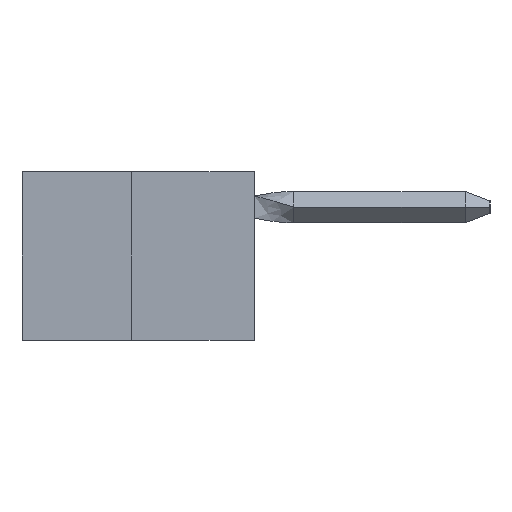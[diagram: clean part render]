
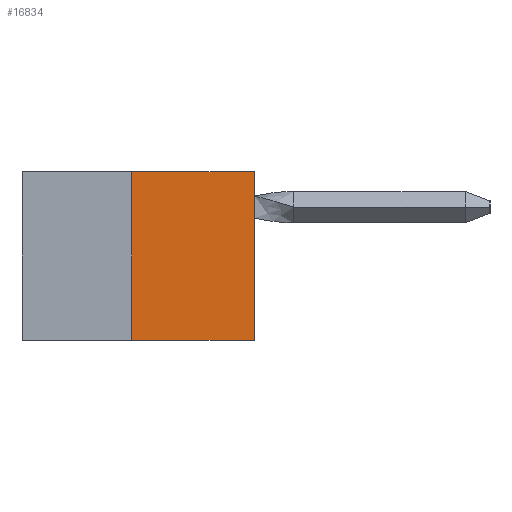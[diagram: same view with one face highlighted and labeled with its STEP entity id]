
A CAD part, left-side view. The second image highlights one B-rep face of the part: STEP entity #16834.
In plain terms, the highlighted planar face has unit normal (-1, 0, 0).
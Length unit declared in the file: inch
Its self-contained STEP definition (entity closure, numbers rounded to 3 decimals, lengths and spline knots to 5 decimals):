
#616 = DIRECTION ( 'NONE',  ( 0., 0., -1. ) ) ;
#1015 = CARTESIAN_POINT ( 'NONE',  ( 0., 0.473, -0.343 ) ) ;
#1435 = VERTEX_POINT ( 'NONE', #10154 ) ;
#1439 = EDGE_CURVE ( 'NONE', #32451, #29499, #21421, .T. ) ;
#4419 = VERTEX_POINT ( 'NONE', #32330 ) ;
#4505 = VECTOR ( 'NONE', #20244, 39.37008 ) ;
#6474 = LINE ( 'NONE', #13407, #26571 ) ;
#6971 = CARTESIAN_POINT ( 'NONE',  ( 0., 0.25, 0. ) ) ;
#7563 = VECTOR ( 'NONE', #35632, 39.37008 ) ;
#8974 = ORIENTED_EDGE ( 'NONE', *, *, #36058, .T. ) ;
#8975 = CARTESIAN_POINT ( 'NONE',  ( 0., 0.473, 0. ) ) ;
#10154 = CARTESIAN_POINT ( 'NONE',  ( 0., 0., 0. ) ) ;
#11006 = LINE ( 'NONE', #1015, #36489 ) ;
#12723 = CARTESIAN_POINT ( 'NONE',  ( 0., 0.25, -0.343 ) ) ;
#13407 = CARTESIAN_POINT ( 'NONE',  ( 0., 0., 0. ) ) ;
#13809 = AXIS2_PLACEMENT_3D ( 'NONE', #8975, #34700, #616 ) ;
#14290 = ORIENTED_EDGE ( 'NONE', *, *, #31448, .T. ) ;
#14759 = CARTESIAN_POINT ( 'NONE',  ( 0., 0.473, 0. ) ) ;
#16834 = ADVANCED_FACE ( 'NONE', ( #19210 ), #29084, .F. ) ;
#19210 = FACE_OUTER_BOUND ( 'NONE', #25173, .T. ) ;
#20244 = DIRECTION ( 'NONE',  ( 0., -1., 0. ) ) ;
#21421 = LINE ( 'NONE', #35746, #7563 ) ;
#21536 = ORIENTED_EDGE ( 'NONE', *, *, #27709, .F. ) ;
#23592 = DIRECTION ( 'NONE',  ( 0., -1., 0. ) ) ;
#25173 = EDGE_LOOP ( 'NONE', ( #21536, #36940, #8974, #14290 ) ) ;
#26571 = VECTOR ( 'NONE', #36392, 39.37008 ) ;
#27709 = EDGE_CURVE ( 'NONE', #29499, #1435, #32191, .T. ) ;
#29084 = PLANE ( 'NONE',  #13809 ) ;
#29499 = VERTEX_POINT ( 'NONE', #6971 ) ;
#31448 = EDGE_CURVE ( 'NONE', #4419, #1435, #6474, .T. ) ;
#32191 = LINE ( 'NONE', #14759, #4505 ) ;
#32330 = CARTESIAN_POINT ( 'NONE',  ( 0., 0., -0.343 ) ) ;
#32451 = VERTEX_POINT ( 'NONE', #12723 ) ;
#34700 = DIRECTION ( 'NONE',  ( 1., 0., 0. ) ) ;
#35632 = DIRECTION ( 'NONE',  ( 0., 0., 1. ) ) ;
#35746 = CARTESIAN_POINT ( 'NONE',  ( 0., 0.25, 0. ) ) ;
#36058 = EDGE_CURVE ( 'NONE', #32451, #4419, #11006, .T. ) ;
#36392 = DIRECTION ( 'NONE',  ( 0., 0., 1. ) ) ;
#36489 = VECTOR ( 'NONE', #23592, 39.37008 ) ;
#36940 = ORIENTED_EDGE ( 'NONE', *, *, #1439, .F. ) ;
